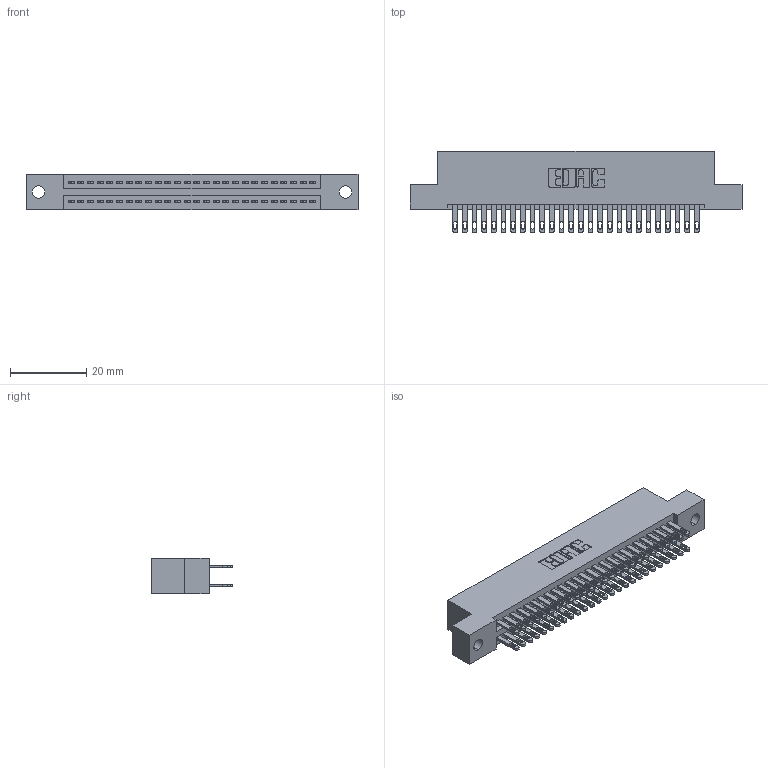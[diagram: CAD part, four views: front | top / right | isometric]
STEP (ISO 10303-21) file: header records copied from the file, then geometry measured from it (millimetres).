
FILE_DESCRIPTION (( 'STEP AP203' ), '1' );
FILE_NAME ('895-052-500-202.STEP', '2020-09-27T10:56:08', ( '' ), ( '' ), 'SwSTEP 2.0', 'SolidWorks 2020', '' );
FILE_SCHEMA (( 'CONFIG_CONTROL_DESIGN' ));
Length unit declared in the file: inch
Products named in the file (3): 895-052-500-202; 345-292-001_345-293-100; 845 Part_Flush Mounting Lugs - 0.128 Dia
Assembly tree (53 placements, depth 2):
  895-052-500-202
    845 Part_Flush Mounting Lugs - 0.128 Dia
    345-292-001_345-293-100  x52
Bounding box: 87.25 x 21.51 x 9.4 mm (x, y, z)
Volume: 8449.2 mm3; surface area: 12437 mm2
Topology: 53 solids, 53 shells, 2518 faces, 7673 edges, 5114 vertices
Faces by surface type: plane 1484, cylinder 1034
Entity records: 22487 total; most frequent: CARTESIAN_POINT 3784, ORIENTED_EDGE 3718, DIRECTION 3359, EDGE_CURVE 1859, LINE 1619, VECTOR 1619, VERTEX_POINT 1238, AXIS2_PLACEMENT_3D 870
